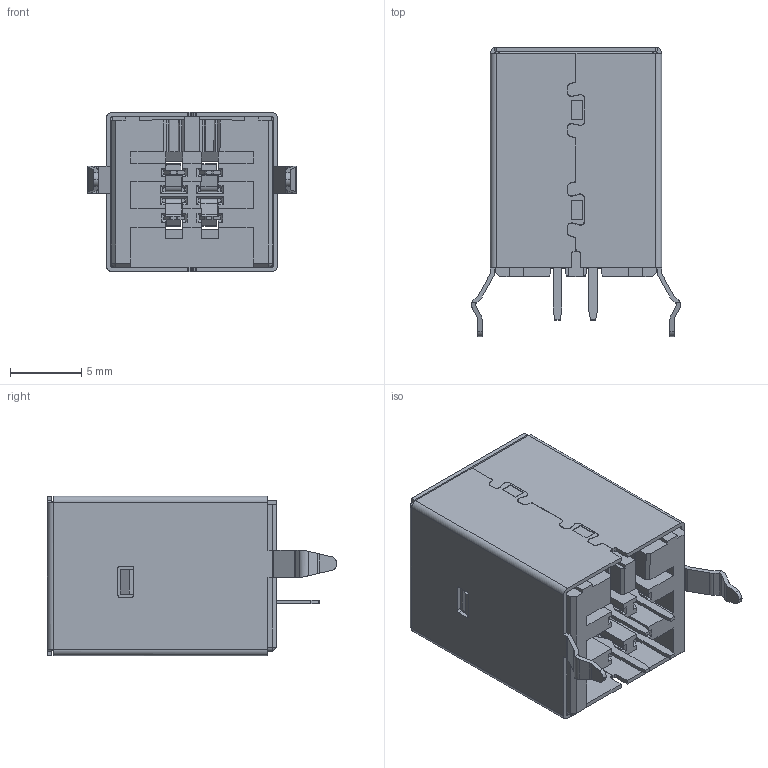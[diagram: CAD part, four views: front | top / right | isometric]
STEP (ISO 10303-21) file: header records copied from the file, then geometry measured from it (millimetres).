
FILE_DESCRIPTION (( 'STEP AP214' ), '1' );
FILE_NAME ('690Q204-143-221.STEP', '2021-01-14T21:23:46', ( '' ), ( '' ), 'SwSTEP 2.0', 'SolidWorks 2020', '' );
FILE_SCHEMA (( 'AUTOMOTIVE_DESIGN' ));
Length unit declared in the file: millimetre
Products named in the file (4): Insulator 690Q204-X43-2XX_Black; Shell 690Q204-X43-2XX; 690Q204-143-221; Contact 690Q204-X43-2XX
Assembly tree (6 placements, depth 2):
  690Q204-143-221
    Insulator 690Q204-X43-2XX_Black
    Contact 690Q204-X43-2XX  x4
    Shell 690Q204-X43-2XX
Bounding box: 14.7 x 20.32 x 11.2 mm (x, y, z)
Volume: 1327.3 mm3; surface area: 3612.2 mm2
Topology: 6 solids, 6 shells, 939 faces, 2689 edges, 1756 vertices
Faces by surface type: plane 698, cylinder 227, cone 12, bspline 2
Entity records: 24390 total; most frequent: CARTESIAN_POINT 6445, ORIENTED_EDGE 4106, DIRECTION 3080, EDGE_CURVE 2053, LINE 1406, VECTOR 1406, VERTEX_POINT 1336, AXIS2_PLACEMENT_3D 837
